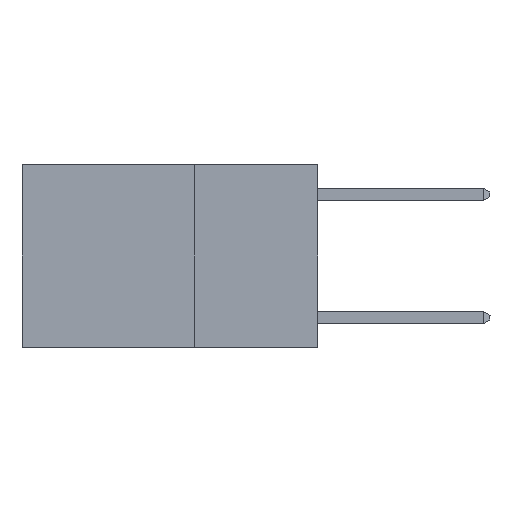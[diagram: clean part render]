
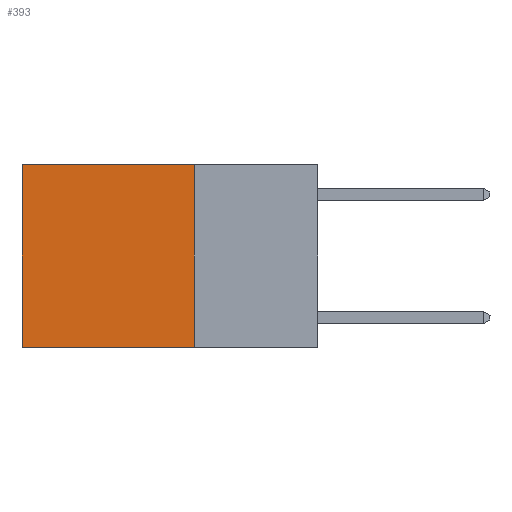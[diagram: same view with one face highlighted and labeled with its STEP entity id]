
A CAD part, left-side view. The second image highlights one B-rep face of the part: STEP entity #393.
In plain terms, the highlighted planar face has unit normal (-1, 0, 0).
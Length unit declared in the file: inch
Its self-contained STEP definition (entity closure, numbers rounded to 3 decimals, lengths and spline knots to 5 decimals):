
#393 = ADVANCED_FACE ( 'NONE', ( #12407 ), #14311, .F. ) ;
#565 = EDGE_CURVE ( 'NONE', #1942, #4958, #12173, .T. ) ;
#1942 = VERTEX_POINT ( 'NONE', #11393 ) ;
#2376 = CARTESIAN_POINT ( 'NONE',  ( 0.2625, 0.25, -0.37 ) ) ;
#2404 = LINE ( 'NONE', #14496, #16659 ) ;
#3832 = DIRECTION ( 'NONE',  ( 0., 1., 0. ) ) ;
#4958 = VERTEX_POINT ( 'NONE', #17496 ) ;
#7838 = VERTEX_POINT ( 'NONE', #13718 ) ;
#8223 = LINE ( 'NONE', #2376, #15275 ) ;
#8857 = VECTOR ( 'NONE', #17067, 39.37008 ) ;
#8915 = AXIS2_PLACEMENT_3D ( 'NONE', #13486, #10907, #10658 ) ;
#10658 = DIRECTION ( 'NONE',  ( 0., 0., -1. ) ) ;
#10813 = EDGE_LOOP ( 'NONE', ( #12850, #12876, #13097, #13729 ) ) ;
#10879 = LINE ( 'NONE', #13294, #14608 ) ;
#10907 = DIRECTION ( 'NONE',  ( 1., 0., 0. ) ) ;
#10919 = EDGE_CURVE ( 'NONE', #7838, #16678, #2404, .T. ) ;
#11393 = CARTESIAN_POINT ( 'NONE',  ( 0.2625, 0.6, 0. ) ) ;
#12048 = CARTESIAN_POINT ( 'NONE',  ( 0.2625, 0.25, -0.37 ) ) ;
#12173 = LINE ( 'NONE', #17229, #8857 ) ;
#12407 = FACE_OUTER_BOUND ( 'NONE', #10813, .T. ) ;
#12850 = ORIENTED_EDGE ( 'NONE', *, *, #565, .T. ) ;
#12876 = ORIENTED_EDGE ( 'NONE', *, *, #15102, .F. ) ;
#13097 = ORIENTED_EDGE ( 'NONE', *, *, #10919, .F. ) ;
#13294 = CARTESIAN_POINT ( 'NONE',  ( 0.2625, 0.25, 0. ) ) ;
#13486 = CARTESIAN_POINT ( 'NONE',  ( 0.2625, 0.25, 0. ) ) ;
#13718 = CARTESIAN_POINT ( 'NONE',  ( 0.2625, 0.25, 0. ) ) ;
#13729 = ORIENTED_EDGE ( 'NONE', *, *, #16571, .T. ) ;
#14311 = PLANE ( 'NONE',  #8915 ) ;
#14496 = CARTESIAN_POINT ( 'NONE',  ( 0.2625, 0.25, 0. ) ) ;
#14608 = VECTOR ( 'NONE', #16063, 39.37008 ) ;
#15102 = EDGE_CURVE ( 'NONE', #16678, #4958, #8223, .T. ) ;
#15275 = VECTOR ( 'NONE', #3832, 39.37008 ) ;
#15851 = DIRECTION ( 'NONE',  ( 0., 0., -1. ) ) ;
#16063 = DIRECTION ( 'NONE',  ( 0., 1., 0. ) ) ;
#16571 = EDGE_CURVE ( 'NONE', #7838, #1942, #10879, .T. ) ;
#16659 = VECTOR ( 'NONE', #15851, 39.37008 ) ;
#16678 = VERTEX_POINT ( 'NONE', #12048 ) ;
#17067 = DIRECTION ( 'NONE',  ( 0., 0., -1. ) ) ;
#17229 = CARTESIAN_POINT ( 'NONE',  ( 0.2625, 0.6, 0. ) ) ;
#17496 = CARTESIAN_POINT ( 'NONE',  ( 0.2625, 0.6, -0.37 ) ) ;
